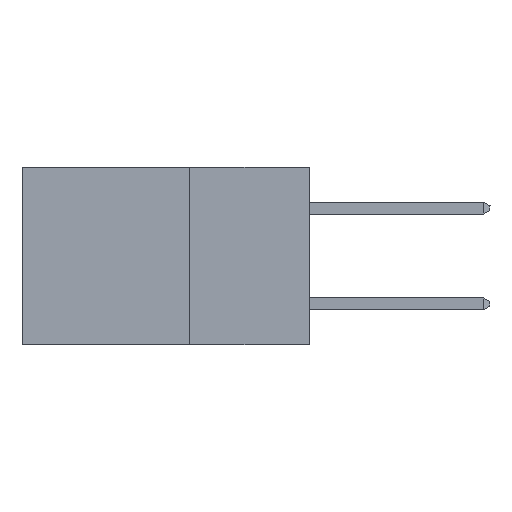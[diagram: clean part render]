
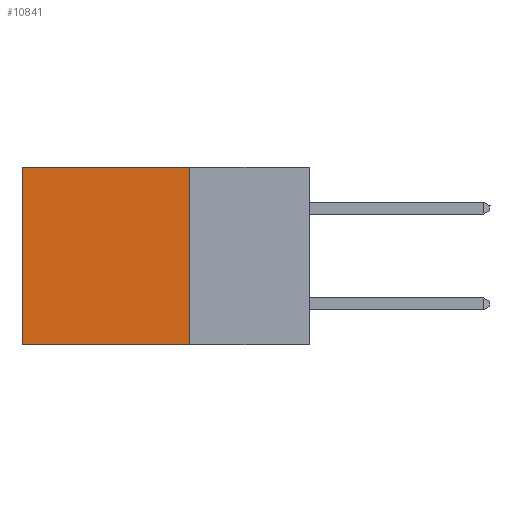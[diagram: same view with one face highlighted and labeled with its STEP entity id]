
A CAD part, left-side view. The second image highlights one B-rep face of the part: STEP entity #10841.
In plain terms, the highlighted planar face has unit normal (-1, 0, 0).
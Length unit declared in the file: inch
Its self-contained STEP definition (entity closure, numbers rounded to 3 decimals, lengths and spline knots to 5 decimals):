
#708 = CARTESIAN_POINT ( 'NONE',  ( 0.2875, 0.25, 0. ) ) ;
#1276 = DIRECTION ( 'NONE',  ( 0., 1., 0. ) ) ;
#3062 = DIRECTION ( 'NONE',  ( 0., 0., -1. ) ) ;
#3217 = CARTESIAN_POINT ( 'NONE',  ( 0.2875, 0.6, 0. ) ) ;
#3313 = EDGE_CURVE ( 'NONE', #11253, #24872, #17191, .T. ) ;
#3755 = CARTESIAN_POINT ( 'NONE',  ( 0.2875, 0.25, 0. ) ) ;
#3776 = VERTEX_POINT ( 'NONE', #21646 ) ;
#5504 = EDGE_LOOP ( 'NONE', ( #29960, #7127, #8052, #27343 ) ) ;
#7127 = ORIENTED_EDGE ( 'NONE', *, *, #20977, .F. ) ;
#7567 = CARTESIAN_POINT ( 'NONE',  ( 0.2875, 0.25, -0.37 ) ) ;
#8052 = ORIENTED_EDGE ( 'NONE', *, *, #20135, .F. ) ;
#10804 = VECTOR ( 'NONE', #3062, 39.37008 ) ;
#10835 = DIRECTION ( 'NONE',  ( 1., 0., 0. ) ) ;
#10841 = ADVANCED_FACE ( 'NONE', ( #26745 ), #23431, .F. ) ;
#11253 = VERTEX_POINT ( 'NONE', #13768 ) ;
#11868 = AXIS2_PLACEMENT_3D ( 'NONE', #708, #10835, #20947 ) ;
#12971 = LINE ( 'NONE', #21081, #27660 ) ;
#13315 = VECTOR ( 'NONE', #18830, 39.37008 ) ;
#13768 = CARTESIAN_POINT ( 'NONE',  ( 0.2875, 0.25, 0. ) ) ;
#17191 = LINE ( 'NONE', #3755, #25348 ) ;
#18091 = DIRECTION ( 'NONE',  ( 0., 1., 0. ) ) ;
#18830 = DIRECTION ( 'NONE',  ( 0., 0., -1. ) ) ;
#20004 = CARTESIAN_POINT ( 'NONE',  ( 0.2875, 0.6, 0. ) ) ;
#20135 = EDGE_CURVE ( 'NONE', #11253, #24856, #28623, .T. ) ;
#20947 = DIRECTION ( 'NONE',  ( 0., 0., -1. ) ) ;
#20977 = EDGE_CURVE ( 'NONE', #24856, #3776, #12971, .T. ) ;
#21081 = CARTESIAN_POINT ( 'NONE',  ( 0.2875, 0.25, -0.37 ) ) ;
#21646 = CARTESIAN_POINT ( 'NONE',  ( 0.2875, 0.6, -0.37 ) ) ;
#23431 = PLANE ( 'NONE',  #11868 ) ;
#24856 = VERTEX_POINT ( 'NONE', #7567 ) ;
#24872 = VERTEX_POINT ( 'NONE', #20004 ) ;
#24955 = EDGE_CURVE ( 'NONE', #24872, #3776, #26126, .T. ) ;
#25348 = VECTOR ( 'NONE', #1276, 39.37008 ) ;
#26126 = LINE ( 'NONE', #3217, #10804 ) ;
#26745 = FACE_OUTER_BOUND ( 'NONE', #5504, .T. ) ;
#27343 = ORIENTED_EDGE ( 'NONE', *, *, #3313, .T. ) ;
#27660 = VECTOR ( 'NONE', #18091, 39.37008 ) ;
#28623 = LINE ( 'NONE', #31440, #13315 ) ;
#29960 = ORIENTED_EDGE ( 'NONE', *, *, #24955, .T. ) ;
#31440 = CARTESIAN_POINT ( 'NONE',  ( 0.2875, 0.25, 0. ) ) ;
